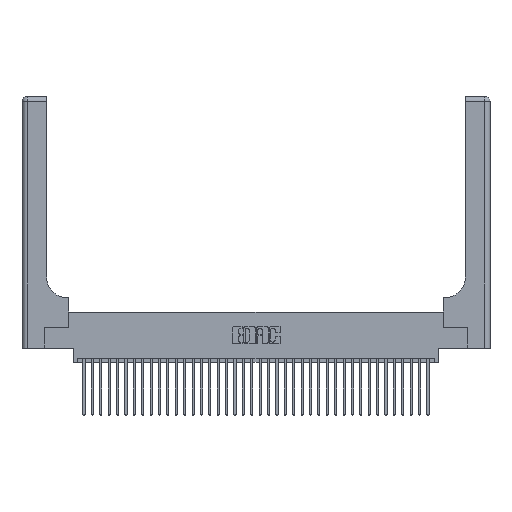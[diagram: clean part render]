
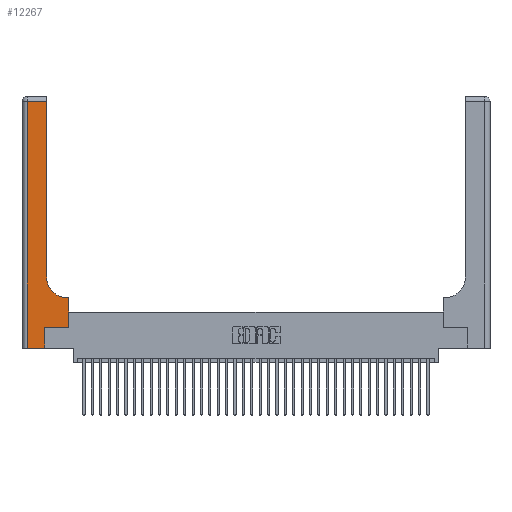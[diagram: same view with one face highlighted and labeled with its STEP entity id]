
A CAD part, top view. The second image highlights one B-rep face of the part: STEP entity #12267.
In plain terms, the highlighted planar face has unit normal (0, 0, 1).
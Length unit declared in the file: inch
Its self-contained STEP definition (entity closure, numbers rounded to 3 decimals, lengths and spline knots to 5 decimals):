
#2115 = ORIENTED_EDGE ( 'NONE', *, *, #21085, .T. ) ;
#2667 = VECTOR ( 'NONE', #20331, 39.37008 ) ;
#3200 = VERTEX_POINT ( 'NONE', #20917 ) ;
#3374 = EDGE_CURVE ( 'NONE', #33159, #29406, #22817, .T. ) ;
#3510 = DIRECTION ( 'NONE',  ( 1., 0., 0. ) ) ;
#3969 = LINE ( 'NONE', #22143, #26667 ) ;
#4072 = DIRECTION ( 'NONE',  ( 0., 1., 0. ) ) ;
#5060 = LINE ( 'NONE', #6601, #37466 ) ;
#5138 = VECTOR ( 'NONE', #36213, 39.37008 ) ;
#5254 = ORIENTED_EDGE ( 'NONE', *, *, #10250, .T. ) ;
#5491 = CIRCLE ( 'NONE', #8883, 0.25 ) ;
#6138 = EDGE_CURVE ( 'NONE', #7385, #33159, #5491, .T. ) ;
#6581 = EDGE_CURVE ( 'NONE', #26515, #3200, #25843, .T. ) ;
#6601 = CARTESIAN_POINT ( 'NONE',  ( 0.269, 0.25, 0.37 ) ) ;
#6971 = CARTESIAN_POINT ( 'NONE',  ( 0.5585, 0.25, 0.37 ) ) ;
#7381 = CARTESIAN_POINT ( 'NONE',  ( 0.2915, 3., 0.37 ) ) ;
#7385 = VERTEX_POINT ( 'NONE', #35060 ) ;
#7633 = ORIENTED_EDGE ( 'NONE', *, *, #3374, .T. ) ;
#7819 = DIRECTION ( 'NONE',  ( 0., 0., -1. ) ) ;
#7888 = VERTEX_POINT ( 'NONE', #18180 ) ;
#7919 = EDGE_CURVE ( 'NONE', #17807, #7385, #33495, .T. ) ;
#8047 = DIRECTION ( 'NONE',  ( 0., 1., 0. ) ) ;
#8883 = AXIS2_PLACEMENT_3D ( 'NONE', #37177, #7819, #13415 ) ;
#9239 = DIRECTION ( 'NONE',  ( 0., 1., 0. ) ) ;
#10072 = EDGE_CURVE ( 'NONE', #3200, #7888, #31498, .T. ) ;
#10250 = EDGE_CURVE ( 'NONE', #37808, #17807, #15243, .T. ) ;
#12073 = ORIENTED_EDGE ( 'NONE', *, *, #6581, .T. ) ;
#12267 = ADVANCED_FACE ( 'NONE', ( #35997 ), #15206, .F. ) ;
#12476 = DIRECTION ( 'NONE',  ( 0., 0., -1. ) ) ;
#13415 = DIRECTION ( 'NONE',  ( 1., 0., 0. ) ) ;
#14570 = CARTESIAN_POINT ( 'NONE',  ( 0.269, 0., 0.37 ) ) ;
#15137 = VERTEX_POINT ( 'NONE', #15628 ) ;
#15206 = PLANE ( 'NONE',  #22126 ) ;
#15243 = LINE ( 'NONE', #6971, #28107 ) ;
#15628 = CARTESIAN_POINT ( 'NONE',  ( 0.269, 0.25, 0.37 ) ) ;
#16597 = DIRECTION ( 'NONE',  ( -1., 0., 0. ) ) ;
#16737 = LINE ( 'NONE', #14570, #31470 ) ;
#16814 = CARTESIAN_POINT ( 'NONE',  ( 0.2915, 2.94, 0.37 ) ) ;
#17535 = ORIENTED_EDGE ( 'NONE', *, *, #28359, .T. ) ;
#17627 = CARTESIAN_POINT ( 'NONE',  ( 0.06, 3., 0.37 ) ) ;
#17694 = CARTESIAN_POINT ( 'NONE',  ( 0.5585, 0.25, 0.37 ) ) ;
#17807 = VERTEX_POINT ( 'NONE', #25852 ) ;
#18180 = CARTESIAN_POINT ( 'NONE',  ( 0.269, 0., 0.37 ) ) ;
#18201 = ORIENTED_EDGE ( 'NONE', *, *, #7919, .T. ) ;
#19243 = EDGE_LOOP ( 'NONE', ( #7633, #21117, #12073, #33280, #2115, #17535, #5254, #18201, #20942 ) ) ;
#20331 = DIRECTION ( 'NONE',  ( 0., -1., 0. ) ) ;
#20826 = CARTESIAN_POINT ( 'NONE',  ( 0.2915, 0.6, 0.37 ) ) ;
#20917 = CARTESIAN_POINT ( 'NONE',  ( 0.06, 0., 0.37 ) ) ;
#20942 = ORIENTED_EDGE ( 'NONE', *, *, #6138, .T. ) ;
#21085 = EDGE_CURVE ( 'NONE', #7888, #15137, #16737, .T. ) ;
#21117 = ORIENTED_EDGE ( 'NONE', *, *, #24745, .T. ) ;
#21137 = CARTESIAN_POINT ( 'NONE',  ( 0.06, 2.94, 0.37 ) ) ;
#21641 = CARTESIAN_POINT ( 'NONE',  ( 0., 3., 0.37 ) ) ;
#22126 = AXIS2_PLACEMENT_3D ( 'NONE', #21641, #12476, #24118 ) ;
#22143 = CARTESIAN_POINT ( 'NONE',  ( 0., 2.94, 0.37 ) ) ;
#22817 = LINE ( 'NONE', #7381, #28786 ) ;
#23855 = VECTOR ( 'NONE', #16597, 39.37008 ) ;
#24118 = DIRECTION ( 'NONE',  ( -1., 0., 0. ) ) ;
#24745 = EDGE_CURVE ( 'NONE', #29406, #26515, #3969, .T. ) ;
#25843 = LINE ( 'NONE', #17627, #2667 ) ;
#25852 = CARTESIAN_POINT ( 'NONE',  ( 0.5585, 0.6, 0.37 ) ) ;
#26515 = VERTEX_POINT ( 'NONE', #21137 ) ;
#26667 = VECTOR ( 'NONE', #28014, 39.37008 ) ;
#28014 = DIRECTION ( 'NONE',  ( -1., 0., 0. ) ) ;
#28107 = VECTOR ( 'NONE', #4072, 39.37008 ) ;
#28359 = EDGE_CURVE ( 'NONE', #15137, #37808, #5060, .T. ) ;
#28786 = VECTOR ( 'NONE', #8047, 39.37008 ) ;
#29406 = VERTEX_POINT ( 'NONE', #16814 ) ;
#31470 = VECTOR ( 'NONE', #9239, 39.37008 ) ;
#31498 = LINE ( 'NONE', #32328, #5138 ) ;
#32328 = CARTESIAN_POINT ( 'NONE',  ( 0., 0., 0.37 ) ) ;
#33159 = VERTEX_POINT ( 'NONE', #38047 ) ;
#33280 = ORIENTED_EDGE ( 'NONE', *, *, #10072, .T. ) ;
#33495 = LINE ( 'NONE', #20826, #23855 ) ;
#35060 = CARTESIAN_POINT ( 'NONE',  ( 0.5415, 0.6, 0.37 ) ) ;
#35997 = FACE_OUTER_BOUND ( 'NONE', #19243, .T. ) ;
#36213 = DIRECTION ( 'NONE',  ( 1., 0., 0. ) ) ;
#37177 = CARTESIAN_POINT ( 'NONE',  ( 0.5415, 0.85, 0.37 ) ) ;
#37466 = VECTOR ( 'NONE', #3510, 39.37008 ) ;
#37808 = VERTEX_POINT ( 'NONE', #17694 ) ;
#38047 = CARTESIAN_POINT ( 'NONE',  ( 0.2915, 0.85, 0.37 ) ) ;
